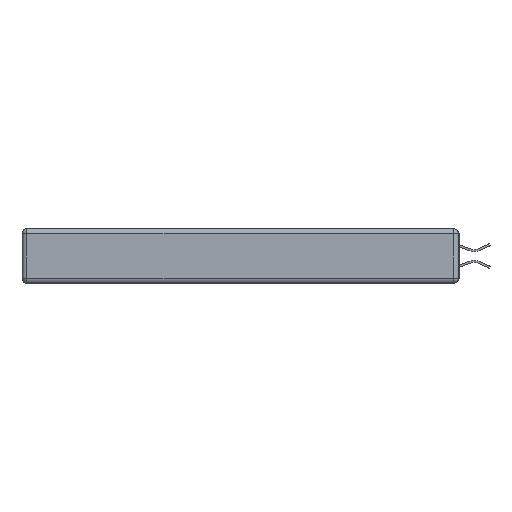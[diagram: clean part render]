
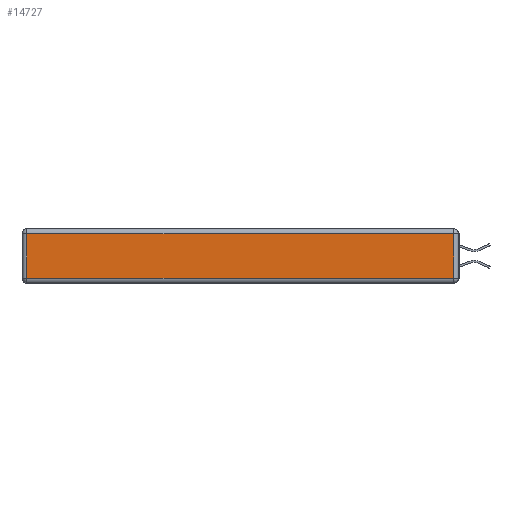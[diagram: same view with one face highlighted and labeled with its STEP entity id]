
A CAD part, left-side view. The second image highlights one B-rep face of the part: STEP entity #14727.
In plain terms, the highlighted planar face has unit normal (-1, 0, 0).
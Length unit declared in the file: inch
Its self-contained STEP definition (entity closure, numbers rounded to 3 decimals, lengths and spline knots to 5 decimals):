
#270 = VERTEX_POINT ( 'NONE', #18812 ) ;
#510 = AXIS2_PLACEMENT_3D ( 'NONE', #746, #3858, #16755 ) ;
#746 = CARTESIAN_POINT ( 'NONE',  ( 0., 0., -0.343 ) ) ;
#1959 = EDGE_CURVE ( 'NONE', #270, #11812, #11837, .T. ) ;
#2111 = DIRECTION ( 'NONE',  ( 0., 0., 1. ) ) ;
#2163 = DIRECTION ( 'NONE',  ( 0., -1., 0. ) ) ;
#3667 = VECTOR ( 'NONE', #15997, 39.37008 ) ;
#3858 = DIRECTION ( 'NONE',  ( -1., 0., 0. ) ) ;
#4782 = VECTOR ( 'NONE', #2111, 39.37008 ) ;
#6953 = CARTESIAN_POINT ( 'NONE',  ( 0., 2.72, -0.03 ) ) ;
#7356 = CARTESIAN_POINT ( 'NONE',  ( 0., 2.75, -0.03 ) ) ;
#8340 = ORIENTED_EDGE ( 'NONE', *, *, #20143, .T. ) ;
#9303 = VECTOR ( 'NONE', #18563, 39.37008 ) ;
#10292 = LINE ( 'NONE', #7356, #9303 ) ;
#10492 = LINE ( 'NONE', #16395, #4782 ) ;
#10853 = EDGE_CURVE ( 'NONE', #15117, #12010, #10292, .T. ) ;
#11085 = FACE_OUTER_BOUND ( 'NONE', #16486, .T. ) ;
#11812 = VERTEX_POINT ( 'NONE', #12477 ) ;
#11837 = LINE ( 'NONE', #13237, #16082 ) ;
#12004 = PLANE ( 'NONE',  #510 ) ;
#12010 = VERTEX_POINT ( 'NONE', #6953 ) ;
#12477 = CARTESIAN_POINT ( 'NONE',  ( 0., 0.03, -0.313 ) ) ;
#12757 = EDGE_CURVE ( 'NONE', #12010, #270, #15306, .T. ) ;
#13237 = CARTESIAN_POINT ( 'NONE',  ( 0., 0., -0.313 ) ) ;
#14208 = CARTESIAN_POINT ( 'NONE',  ( 0., 2.72, -0.343 ) ) ;
#14727 = ADVANCED_FACE ( 'NONE', ( #11085 ), #12004, .T. ) ;
#15117 = VERTEX_POINT ( 'NONE', #15724 ) ;
#15306 = LINE ( 'NONE', #14208, #3667 ) ;
#15724 = CARTESIAN_POINT ( 'NONE',  ( 0., 0.03, -0.03 ) ) ;
#15997 = DIRECTION ( 'NONE',  ( 0., 0., -1. ) ) ;
#16082 = VECTOR ( 'NONE', #2163, 39.37008 ) ;
#16395 = CARTESIAN_POINT ( 'NONE',  ( 0., 0.03, -0.343 ) ) ;
#16486 = EDGE_LOOP ( 'NONE', ( #18506, #8340, #20384, #20035 ) ) ;
#16755 = DIRECTION ( 'NONE',  ( 0., 0., 1. ) ) ;
#18506 = ORIENTED_EDGE ( 'NONE', *, *, #1959, .T. ) ;
#18563 = DIRECTION ( 'NONE',  ( 0., 1., 0. ) ) ;
#18812 = CARTESIAN_POINT ( 'NONE',  ( 0., 2.72, -0.313 ) ) ;
#20035 = ORIENTED_EDGE ( 'NONE', *, *, #12757, .T. ) ;
#20143 = EDGE_CURVE ( 'NONE', #11812, #15117, #10492, .T. ) ;
#20384 = ORIENTED_EDGE ( 'NONE', *, *, #10853, .T. ) ;
